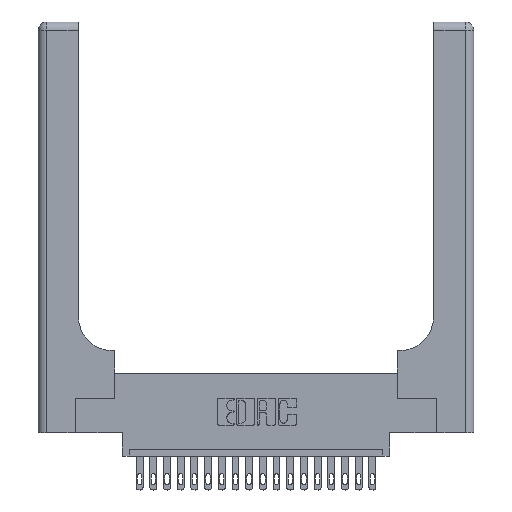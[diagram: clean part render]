
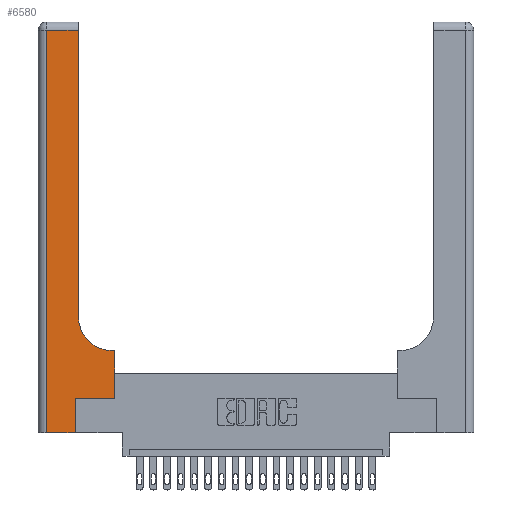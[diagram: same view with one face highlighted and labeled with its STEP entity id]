
A CAD part, top view. The second image highlights one B-rep face of the part: STEP entity #6580.
In plain terms, the highlighted planar face has unit normal (0, 0, 1).
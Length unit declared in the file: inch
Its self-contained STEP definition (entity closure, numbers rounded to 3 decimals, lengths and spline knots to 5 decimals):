
#85 = EDGE_CURVE ( 'NONE', #17221, #8744, #18109, .T. ) ;
#349 = CARTESIAN_POINT ( 'NONE',  ( 0.06, 2.94, 0.37 ) ) ;
#418 = CARTESIAN_POINT ( 'NONE',  ( 0.06, 0., 0.37 ) ) ;
#531 = LINE ( 'NONE', #2601, #1362 ) ;
#557 = ORIENTED_EDGE ( 'NONE', *, *, #2440, .T. ) ;
#675 = PLANE ( 'NONE',  #14875 ) ;
#1167 = DIRECTION ( 'NONE',  ( -1., 0., 0. ) ) ;
#1348 = VECTOR ( 'NONE', #6125, 39.37008 ) ;
#1362 = VECTOR ( 'NONE', #4143, 39.37008 ) ;
#1425 = ORIENTED_EDGE ( 'NONE', *, *, #18205, .T. ) ;
#1538 = DIRECTION ( 'NONE',  ( 1., 0., 0. ) ) ;
#1618 = EDGE_CURVE ( 'NONE', #7736, #17146, #7941, .T. ) ;
#2440 = EDGE_CURVE ( 'NONE', #6712, #9630, #16931, .T. ) ;
#2601 = CARTESIAN_POINT ( 'NONE',  ( 0.269, 0., 0.37 ) ) ;
#2730 = CARTESIAN_POINT ( 'NONE',  ( 0., 0., 0.37 ) ) ;
#3419 = CARTESIAN_POINT ( 'NONE',  ( 0.5585, 0.6, 0.37 ) ) ;
#3789 = EDGE_CURVE ( 'NONE', #12746, #6712, #5850, .T. ) ;
#4143 = DIRECTION ( 'NONE',  ( 0., 1., 0. ) ) ;
#4171 = DIRECTION ( 'NONE',  ( -1., 0., 0. ) ) ;
#4353 = VECTOR ( 'NONE', #21018, 39.37008 ) ;
#4654 = DIRECTION ( 'NONE',  ( 0., 1., 0. ) ) ;
#5303 = EDGE_CURVE ( 'NONE', #9630, #8729, #8860, .T. ) ;
#5591 = CARTESIAN_POINT ( 'NONE',  ( 0.269, 0., 0.37 ) ) ;
#5694 = CIRCLE ( 'NONE', #6235, 0.25 ) ;
#5850 = LINE ( 'NONE', #7785, #1348 ) ;
#5918 = CARTESIAN_POINT ( 'NONE',  ( 0.2915, 0.85, 0.37 ) ) ;
#6125 = DIRECTION ( 'NONE',  ( 1., 0., 0. ) ) ;
#6157 = DIRECTION ( 'NONE',  ( 0., -1., 0. ) ) ;
#6235 = AXIS2_PLACEMENT_3D ( 'NONE', #18385, #8213, #1538 ) ;
#6580 = ADVANCED_FACE ( 'NONE', ( #20761 ), #675, .F. ) ;
#6712 = VERTEX_POINT ( 'NONE', #11039 ) ;
#7006 = EDGE_CURVE ( 'NONE', #12038, #12746, #531, .T. ) ;
#7415 = ORIENTED_EDGE ( 'NONE', *, *, #5303, .T. ) ;
#7736 = VERTEX_POINT ( 'NONE', #349 ) ;
#7785 = CARTESIAN_POINT ( 'NONE',  ( 0.269, 0.25, 0.37 ) ) ;
#7941 = LINE ( 'NONE', #16485, #9556 ) ;
#8213 = DIRECTION ( 'NONE',  ( 0., 0., -1. ) ) ;
#8495 = ORIENTED_EDGE ( 'NONE', *, *, #16163, .T. ) ;
#8683 = ORIENTED_EDGE ( 'NONE', *, *, #9995, .T. ) ;
#8729 = VERTEX_POINT ( 'NONE', #10489 ) ;
#8744 = VERTEX_POINT ( 'NONE', #13990 ) ;
#8860 = LINE ( 'NONE', #12649, #4353 ) ;
#9556 = VECTOR ( 'NONE', #6157, 39.37008 ) ;
#9630 = VERTEX_POINT ( 'NONE', #3419 ) ;
#9995 = EDGE_CURVE ( 'NONE', #8744, #7736, #15325, .T. ) ;
#10029 = ORIENTED_EDGE ( 'NONE', *, *, #1618, .T. ) ;
#10489 = CARTESIAN_POINT ( 'NONE',  ( 0.5415, 0.6, 0.37 ) ) ;
#11035 = CARTESIAN_POINT ( 'NONE',  ( 0.2915, 3., 0.37 ) ) ;
#11039 = CARTESIAN_POINT ( 'NONE',  ( 0.5585, 0.25, 0.37 ) ) ;
#11334 = VECTOR ( 'NONE', #1167, 39.37008 ) ;
#12038 = VERTEX_POINT ( 'NONE', #5591 ) ;
#12444 = VECTOR ( 'NONE', #18880, 39.37008 ) ;
#12517 = DIRECTION ( 'NONE',  ( 0., 0., -1. ) ) ;
#12649 = CARTESIAN_POINT ( 'NONE',  ( 0.2915, 0.6, 0.37 ) ) ;
#12746 = VERTEX_POINT ( 'NONE', #16685 ) ;
#13442 = VECTOR ( 'NONE', #18013, 39.37008 ) ;
#13922 = CARTESIAN_POINT ( 'NONE',  ( 0.5585, 0.25, 0.37 ) ) ;
#13990 = CARTESIAN_POINT ( 'NONE',  ( 0.2915, 2.94, 0.37 ) ) ;
#14496 = LINE ( 'NONE', #2730, #13442 ) ;
#14826 = ORIENTED_EDGE ( 'NONE', *, *, #85, .T. ) ;
#14875 = AXIS2_PLACEMENT_3D ( 'NONE', #15982, #12517, #4171 ) ;
#15325 = LINE ( 'NONE', #19725, #11334 ) ;
#15442 = VECTOR ( 'NONE', #4654, 39.37008 ) ;
#15982 = CARTESIAN_POINT ( 'NONE',  ( 0., 3., 0.37 ) ) ;
#16163 = EDGE_CURVE ( 'NONE', #17146, #12038, #14496, .T. ) ;
#16485 = CARTESIAN_POINT ( 'NONE',  ( 0.06, 3., 0.37 ) ) ;
#16685 = CARTESIAN_POINT ( 'NONE',  ( 0.269, 0.25, 0.37 ) ) ;
#16931 = LINE ( 'NONE', #13922, #12444 ) ;
#17146 = VERTEX_POINT ( 'NONE', #418 ) ;
#17221 = VERTEX_POINT ( 'NONE', #5918 ) ;
#17365 = ORIENTED_EDGE ( 'NONE', *, *, #3789, .T. ) ;
#18013 = DIRECTION ( 'NONE',  ( 1., 0., 0. ) ) ;
#18109 = LINE ( 'NONE', #11035, #15442 ) ;
#18205 = EDGE_CURVE ( 'NONE', #8729, #17221, #5694, .T. ) ;
#18385 = CARTESIAN_POINT ( 'NONE',  ( 0.5415, 0.85, 0.37 ) ) ;
#18880 = DIRECTION ( 'NONE',  ( 0., 1., 0. ) ) ;
#19404 = ORIENTED_EDGE ( 'NONE', *, *, #7006, .T. ) ;
#19725 = CARTESIAN_POINT ( 'NONE',  ( 0., 2.94, 0.37 ) ) ;
#20298 = EDGE_LOOP ( 'NONE', ( #14826, #8683, #10029, #8495, #19404, #17365, #557, #7415, #1425 ) ) ;
#20761 = FACE_OUTER_BOUND ( 'NONE', #20298, .T. ) ;
#21018 = DIRECTION ( 'NONE',  ( -1., 0., 0. ) ) ;
